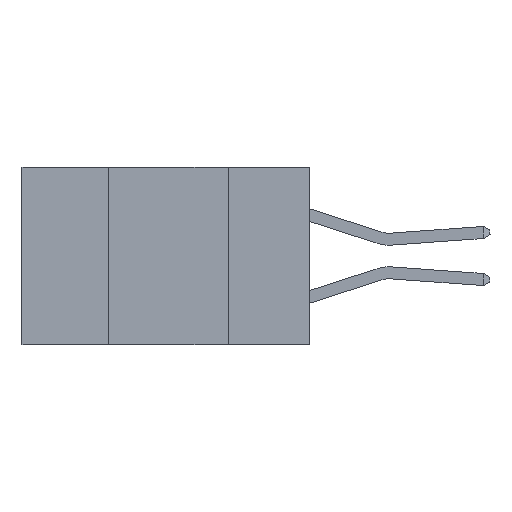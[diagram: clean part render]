
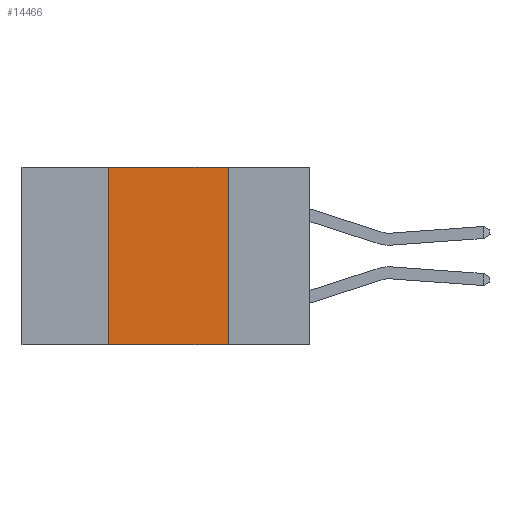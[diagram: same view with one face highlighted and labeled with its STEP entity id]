
A CAD part, left-side view. The second image highlights one B-rep face of the part: STEP entity #14466.
In plain terms, the highlighted planar face has unit normal (-1, 0, 0).
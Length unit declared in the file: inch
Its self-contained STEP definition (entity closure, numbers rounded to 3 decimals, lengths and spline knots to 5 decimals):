
#122 = DIRECTION ( 'NONE',  ( 0., 0., 1. ) ) ;
#177 = LINE ( 'NONE', #6962, #4809 ) ;
#180 = DIRECTION ( 'NONE',  ( 0., 0., -1. ) ) ;
#619 = VECTOR ( 'NONE', #10900, 39.37008 ) ;
#1185 = FACE_OUTER_BOUND ( 'NONE', #14285, .T. ) ;
#1965 = CARTESIAN_POINT ( 'NONE',  ( 0., 0.17, -0.37 ) ) ;
#3684 = ORIENTED_EDGE ( 'NONE', *, *, #8148, .F. ) ;
#4809 = VECTOR ( 'NONE', #10965, 39.37008 ) ;
#5275 = ORIENTED_EDGE ( 'NONE', *, *, #6640, .F. ) ;
#5276 = ORIENTED_EDGE ( 'NONE', *, *, #6126, .T. ) ;
#6126 = EDGE_CURVE ( 'NONE', #14237, #10668, #12677, .T. ) ;
#6640 = EDGE_CURVE ( 'NONE', #7363, #10668, #177, .T. ) ;
#6888 = PLANE ( 'NONE',  #11676 ) ;
#6962 = CARTESIAN_POINT ( 'NONE',  ( 0., 0.17, -0.37 ) ) ;
#7253 = CARTESIAN_POINT ( 'NONE',  ( 0., 0.6, -0.37 ) ) ;
#7363 = VERTEX_POINT ( 'NONE', #14650 ) ;
#8148 = EDGE_CURVE ( 'NONE', #15694, #7363, #14817, .T. ) ;
#8253 = VECTOR ( 'NONE', #10989, 39.37008 ) ;
#8296 = CARTESIAN_POINT ( 'NONE',  ( 0., 0.6, 0. ) ) ;
#8845 = VECTOR ( 'NONE', #122, 39.37008 ) ;
#9646 = CARTESIAN_POINT ( 'NONE',  ( 0., 0.6, 0. ) ) ;
#10361 = CARTESIAN_POINT ( 'NONE',  ( 0., 0.42, -0.37 ) ) ;
#10668 = VERTEX_POINT ( 'NONE', #1965 ) ;
#10900 = DIRECTION ( 'NONE',  ( 0., -1., 0. ) ) ;
#10965 = DIRECTION ( 'NONE',  ( 0., 0., -1. ) ) ;
#10989 = DIRECTION ( 'NONE',  ( 0., -1., 0. ) ) ;
#11676 = AXIS2_PLACEMENT_3D ( 'NONE', #8296, #12317, #180 ) ;
#12317 = DIRECTION ( 'NONE',  ( 1., 0., 0. ) ) ;
#12677 = LINE ( 'NONE', #7253, #8253 ) ;
#12776 = CARTESIAN_POINT ( 'NONE',  ( 0., 0.42, 0. ) ) ;
#13234 = LINE ( 'NONE', #17320, #8845 ) ;
#14237 = VERTEX_POINT ( 'NONE', #10361 ) ;
#14285 = EDGE_LOOP ( 'NONE', ( #5275, #3684, #14443, #5276 ) ) ;
#14443 = ORIENTED_EDGE ( 'NONE', *, *, #16047, .F. ) ;
#14466 = ADVANCED_FACE ( 'NONE', ( #1185 ), #6888, .F. ) ;
#14650 = CARTESIAN_POINT ( 'NONE',  ( 0., 0.17, 0. ) ) ;
#14817 = LINE ( 'NONE', #9646, #619 ) ;
#15694 = VERTEX_POINT ( 'NONE', #12776 ) ;
#16047 = EDGE_CURVE ( 'NONE', #14237, #15694, #13234, .T. ) ;
#17320 = CARTESIAN_POINT ( 'NONE',  ( 0., 0.42, -0.37 ) ) ;
